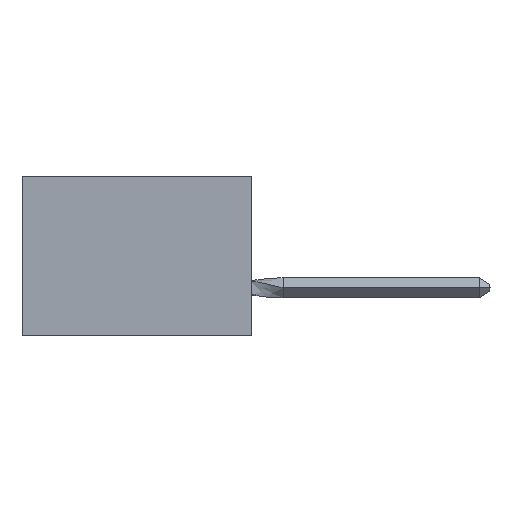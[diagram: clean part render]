
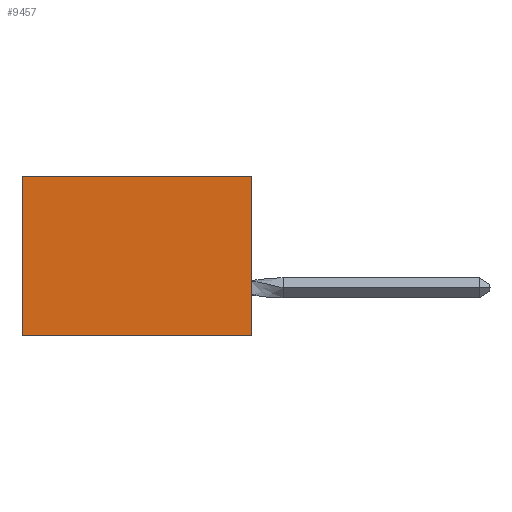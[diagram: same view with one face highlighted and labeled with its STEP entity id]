
A CAD part, left-side view. The second image highlights one B-rep face of the part: STEP entity #9457.
In plain terms, the highlighted planar face has unit normal (-1, 0, 0).
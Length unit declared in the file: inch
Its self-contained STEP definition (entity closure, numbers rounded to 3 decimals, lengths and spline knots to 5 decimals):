
#687 = ORIENTED_EDGE ( 'NONE', *, *, #16817, .T. ) ;
#1904 = VECTOR ( 'NONE', #18537, 39.37008 ) ;
#2793 = PLANE ( 'NONE',  #3505 ) ;
#3505 = AXIS2_PLACEMENT_3D ( 'NONE', #16823, #9896, #7584 ) ;
#6971 = CARTESIAN_POINT ( 'NONE',  ( 0.305, 0.72, -0.5 ) ) ;
#7584 = DIRECTION ( 'NONE',  ( 0., 0., -1. ) ) ;
#8164 = ORIENTED_EDGE ( 'NONE', *, *, #27540, .F. ) ;
#9256 = LINE ( 'NONE', #21844, #16158 ) ;
#9457 = ADVANCED_FACE ( 'NONE', ( #28436 ), #2793, .F. ) ;
#9896 = DIRECTION ( 'NONE',  ( 1., 0., 0. ) ) ;
#10387 = DIRECTION ( 'NONE',  ( 0., 1., 0. ) ) ;
#10437 = LINE ( 'NONE', #21166, #14092 ) ;
#11002 = DIRECTION ( 'NONE',  ( 0., 1., 0. ) ) ;
#11959 = DIRECTION ( 'NONE',  ( 0., 0., -1. ) ) ;
#13958 = CARTESIAN_POINT ( 'NONE',  ( 0.305, 0., 0. ) ) ;
#14092 = VECTOR ( 'NONE', #11959, 39.37008 ) ;
#14111 = ORIENTED_EDGE ( 'NONE', *, *, #20488, .T. ) ;
#15267 = LINE ( 'NONE', #16107, #1904 ) ;
#16107 = CARTESIAN_POINT ( 'NONE',  ( 0.305, 0.72, -0.5 ) ) ;
#16158 = VECTOR ( 'NONE', #11002, 39.37008 ) ;
#16817 = EDGE_CURVE ( 'NONE', #27625, #23315, #15267, .T. ) ;
#16823 = CARTESIAN_POINT ( 'NONE',  ( 0.305, 0., -0.5 ) ) ;
#18537 = DIRECTION ( 'NONE',  ( 0., 0., -1. ) ) ;
#19192 = CARTESIAN_POINT ( 'NONE',  ( 0.305, 0., -0.5 ) ) ;
#20237 = LINE ( 'NONE', #22058, #24894 ) ;
#20488 = EDGE_CURVE ( 'NONE', #23426, #27625, #9256, .T. ) ;
#21166 = CARTESIAN_POINT ( 'NONE',  ( 0.305, 0., -0.5 ) ) ;
#21270 = CARTESIAN_POINT ( 'NONE',  ( 0.305, 0.72, 0. ) ) ;
#21844 = CARTESIAN_POINT ( 'NONE',  ( 0.305, 0., 0. ) ) ;
#22058 = CARTESIAN_POINT ( 'NONE',  ( 0.305, 0., -0.5 ) ) ;
#22374 = ORIENTED_EDGE ( 'NONE', *, *, #27808, .F. ) ;
#22771 = VERTEX_POINT ( 'NONE', #19192 ) ;
#23315 = VERTEX_POINT ( 'NONE', #6971 ) ;
#23426 = VERTEX_POINT ( 'NONE', #13958 ) ;
#24894 = VECTOR ( 'NONE', #10387, 39.37008 ) ;
#27540 = EDGE_CURVE ( 'NONE', #23426, #22771, #10437, .T. ) ;
#27625 = VERTEX_POINT ( 'NONE', #21270 ) ;
#27808 = EDGE_CURVE ( 'NONE', #22771, #23315, #20237, .T. ) ;
#28436 = FACE_OUTER_BOUND ( 'NONE', #29212, .T. ) ;
#29212 = EDGE_LOOP ( 'NONE', ( #687, #22374, #8164, #14111 ) ) ;
